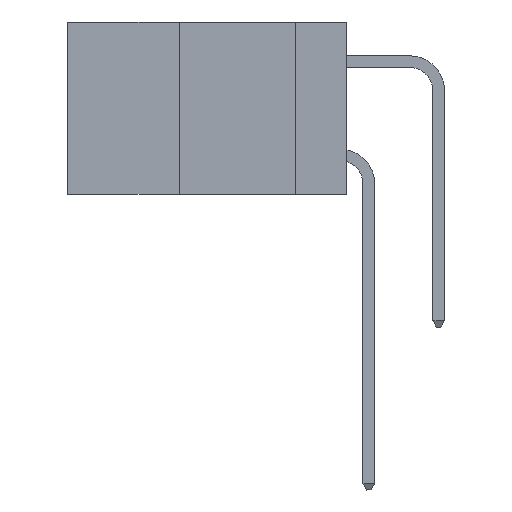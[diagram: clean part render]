
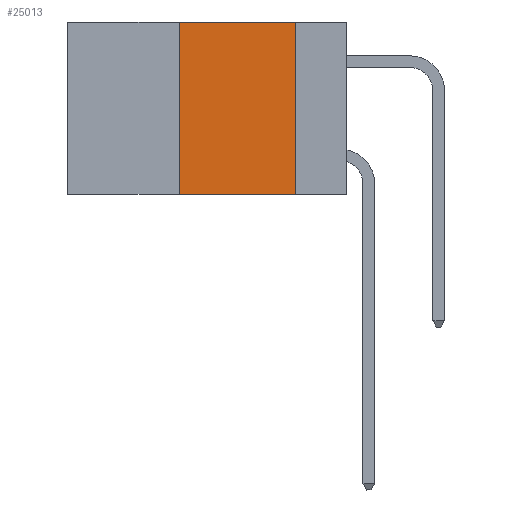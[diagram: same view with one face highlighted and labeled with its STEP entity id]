
A CAD part, left-side view. The second image highlights one B-rep face of the part: STEP entity #25013.
In plain terms, the highlighted planar face has unit normal (-1, 0, 0).
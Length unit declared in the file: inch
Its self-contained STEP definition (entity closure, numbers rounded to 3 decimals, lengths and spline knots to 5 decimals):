
#514 = DIRECTION ( 'NONE',  ( 0., 0., 1. ) ) ;
#1307 = LINE ( 'NONE', #21057, #25208 ) ;
#4217 = PLANE ( 'NONE',  #26492 ) ;
#4654 = DIRECTION ( 'NONE',  ( 0., 0., -1. ) ) ;
#5157 = ORIENTED_EDGE ( 'NONE', *, *, #9279, .F. ) ;
#5966 = VERTEX_POINT ( 'NONE', #9878 ) ;
#6176 = VERTEX_POINT ( 'NONE', #17278 ) ;
#6189 = CARTESIAN_POINT ( 'NONE',  ( 0., 0.36, 0. ) ) ;
#6629 = CARTESIAN_POINT ( 'NONE',  ( 0., 0.6, -0.37 ) ) ;
#6725 = CARTESIAN_POINT ( 'NONE',  ( 0., 0.36, 0. ) ) ;
#9279 = EDGE_CURVE ( 'NONE', #5966, #6176, #1307, .T. ) ;
#9806 = EDGE_CURVE ( 'NONE', #20009, #9968, #26088, .T. ) ;
#9878 = CARTESIAN_POINT ( 'NONE',  ( 0., 0.11, 0. ) ) ;
#9968 = VERTEX_POINT ( 'NONE', #6725 ) ;
#11835 = VECTOR ( 'NONE', #24341, 39.37008 ) ;
#12286 = DIRECTION ( 'NONE',  ( 0., 0., -1. ) ) ;
#13785 = CARTESIAN_POINT ( 'NONE',  ( 0., 0.6, 0. ) ) ;
#15170 = EDGE_CURVE ( 'NONE', #9968, #5966, #15836, .T. ) ;
#15499 = CARTESIAN_POINT ( 'NONE',  ( 0., 0.6, 0. ) ) ;
#15836 = LINE ( 'NONE', #13785, #25269 ) ;
#15986 = EDGE_CURVE ( 'NONE', #20009, #6176, #22042, .T. ) ;
#17278 = CARTESIAN_POINT ( 'NONE',  ( 0., 0.11, -0.37 ) ) ;
#17477 = VECTOR ( 'NONE', #514, 39.37008 ) ;
#19520 = ORIENTED_EDGE ( 'NONE', *, *, #15170, .F. ) ;
#19883 = ORIENTED_EDGE ( 'NONE', *, *, #9806, .F. ) ;
#20009 = VERTEX_POINT ( 'NONE', #26826 ) ;
#21057 = CARTESIAN_POINT ( 'NONE',  ( 0., 0.11, 0. ) ) ;
#21172 = EDGE_LOOP ( 'NONE', ( #5157, #19520, #19883, #21786 ) ) ;
#21786 = ORIENTED_EDGE ( 'NONE', *, *, #15986, .T. ) ;
#22042 = LINE ( 'NONE', #6629, #11835 ) ;
#22697 = DIRECTION ( 'NONE',  ( 0., -1., 0. ) ) ;
#24341 = DIRECTION ( 'NONE',  ( 0., -1., 0. ) ) ;
#25013 = ADVANCED_FACE ( 'NONE', ( #26887 ), #4217, .F. ) ;
#25208 = VECTOR ( 'NONE', #12286, 39.37008 ) ;
#25269 = VECTOR ( 'NONE', #22697, 39.37008 ) ;
#26088 = LINE ( 'NONE', #6189, #17477 ) ;
#26282 = DIRECTION ( 'NONE',  ( 1., 0., 0. ) ) ;
#26492 = AXIS2_PLACEMENT_3D ( 'NONE', #15499, #26282, #4654 ) ;
#26826 = CARTESIAN_POINT ( 'NONE',  ( 0., 0.36, -0.37 ) ) ;
#26887 = FACE_OUTER_BOUND ( 'NONE', #21172, .T. ) ;
